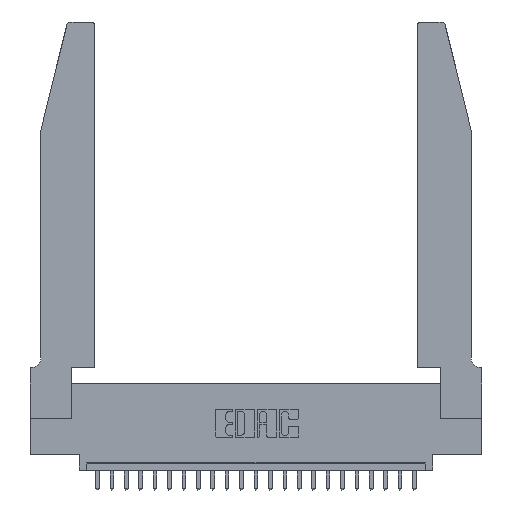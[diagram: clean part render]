
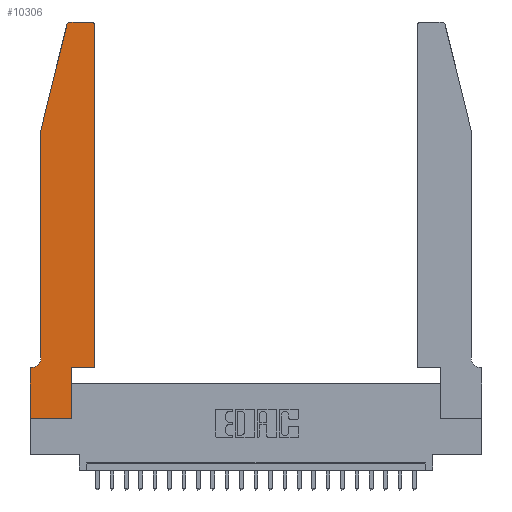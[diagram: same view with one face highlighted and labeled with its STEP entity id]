
A CAD part, top view. The second image highlights one B-rep face of the part: STEP entity #10306.
In plain terms, the highlighted planar face has unit normal (0, 0, 1).
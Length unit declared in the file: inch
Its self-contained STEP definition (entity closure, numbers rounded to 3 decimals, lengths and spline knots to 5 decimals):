
#1007 = CIRCLE ( 'NONE', #1622, 0.03 ) ;
#1274 = CARTESIAN_POINT ( 'NONE',  ( 0.4505, 0.35, 0.37 ) ) ;
#1544 = DIRECTION ( 'NONE',  ( 0., 0., 1. ) ) ;
#1580 = VECTOR ( 'NONE', #18417, 39.37008 ) ;
#1622 = AXIS2_PLACEMENT_3D ( 'NONE', #13395, #7715, #19280 ) ;
#1625 = DIRECTION ( 'NONE',  ( 1., 0., 0. ) ) ;
#1990 = ORIENTED_EDGE ( 'NONE', *, *, #8757, .T. ) ;
#2129 = LINE ( 'NONE', #23747, #23075 ) ;
#2935 = ORIENTED_EDGE ( 'NONE', *, *, #4413, .T. ) ;
#3007 = EDGE_CURVE ( 'NONE', #4921, #15804, #4898, .T. ) ;
#3213 = CARTESIAN_POINT ( 'NONE',  ( 0., 0., 0.37 ) ) ;
#3584 = CARTESIAN_POINT ( 'NONE',  ( 0.284, 2.72, 0.37 ) ) ;
#3932 = VERTEX_POINT ( 'NONE', #20603 ) ;
#4021 = VERTEX_POINT ( 'NONE', #6823 ) ;
#4277 = EDGE_CURVE ( 'NONE', #3932, #5333, #21621, .T. ) ;
#4413 = EDGE_CURVE ( 'NONE', #14375, #3932, #19214, .T. ) ;
#4443 = CARTESIAN_POINT ( 'NONE',  ( 0.0055, 0.35, 0.37 ) ) ;
#4565 = VECTOR ( 'NONE', #5075, 39.37008 ) ;
#4867 = VERTEX_POINT ( 'NONE', #18776 ) ;
#4884 = EDGE_CURVE ( 'NONE', #12663, #22410, #17072, .T. ) ;
#4898 = LINE ( 'NONE', #14768, #4565 ) ;
#4921 = VERTEX_POINT ( 'NONE', #5695 ) ;
#5075 = DIRECTION ( 'NONE',  ( 0., -1., 0. ) ) ;
#5246 = DIRECTION ( 'NONE',  ( 0., 0., -1. ) ) ;
#5313 = EDGE_CURVE ( 'NONE', #5333, #4921, #2129, .T. ) ;
#5333 = VERTEX_POINT ( 'NONE', #9057 ) ;
#5490 = VERTEX_POINT ( 'NONE', #4443 ) ;
#5508 = CARTESIAN_POINT ( 'NONE',  ( 0., 0., 0.37 ) ) ;
#5695 = CARTESIAN_POINT ( 'NONE',  ( 0.0755, 2., 0.37 ) ) ;
#5872 = LINE ( 'NONE', #5508, #15428 ) ;
#6413 = LINE ( 'NONE', #1274, #12709 ) ;
#6823 = CARTESIAN_POINT ( 'NONE',  ( 0.2865, 0.35, 0.37 ) ) ;
#7454 = DIRECTION ( 'NONE',  ( 0., 0., 1. ) ) ;
#7471 = PLANE ( 'NONE',  #10209 ) ;
#7536 = CARTESIAN_POINT ( 'NONE',  ( 0.4505, 0.35, 0.37 ) ) ;
#7715 = DIRECTION ( 'NONE',  ( 0., 0., 1. ) ) ;
#7973 = ORIENTED_EDGE ( 'NONE', *, *, #13818, .T. ) ;
#8038 = CARTESIAN_POINT ( 'NONE',  ( 0.0755, 0.35, 0.37 ) ) ;
#8757 = EDGE_CURVE ( 'NONE', #15804, #5490, #24688, .T. ) ;
#9057 = CARTESIAN_POINT ( 'NONE',  ( 0.25487, 2.72718, 0.37 ) ) ;
#9566 = DIRECTION ( 'NONE',  ( -1., 0., 0. ) ) ;
#10193 = LINE ( 'NONE', #7536, #18278 ) ;
#10209 = AXIS2_PLACEMENT_3D ( 'NONE', #15140, #1544, #1625 ) ;
#10306 = ADVANCED_FACE ( 'NONE', ( #22839 ), #7471, .T. ) ;
#10510 = CARTESIAN_POINT ( 'NONE',  ( 0., 0.35, 0.37 ) ) ;
#10618 = EDGE_CURVE ( 'NONE', #22410, #4021, #22213, .T. ) ;
#10808 = VECTOR ( 'NONE', #9566, 39.37008 ) ;
#11042 = ORIENTED_EDGE ( 'NONE', *, *, #4884, .T. ) ;
#11117 = DIRECTION ( 'NONE',  ( 1., 0., 0. ) ) ;
#11588 = ORIENTED_EDGE ( 'NONE', *, *, #4277, .T. ) ;
#11668 = ORIENTED_EDGE ( 'NONE', *, *, #22695, .T. ) ;
#12079 = VERTEX_POINT ( 'NONE', #10510 ) ;
#12152 = CARTESIAN_POINT ( 'NONE',  ( 0., 0., 0.37 ) ) ;
#12483 = CARTESIAN_POINT ( 'NONE',  ( 0.2865, 0., 0.37 ) ) ;
#12663 = VERTEX_POINT ( 'NONE', #12152 ) ;
#12709 = VECTOR ( 'NONE', #16323, 39.37008 ) ;
#12897 = CARTESIAN_POINT ( 'NONE',  ( 0.4505, 0.35, 0.37 ) ) ;
#13355 = EDGE_LOOP ( 'NONE', ( #2935, #11588, #17117, #16468, #1990, #20863, #7973, #11042, #15535, #14066, #24223, #11668 ) ) ;
#13394 = VERTEX_POINT ( 'NONE', #12897 ) ;
#13395 = CARTESIAN_POINT ( 'NONE',  ( 0.4205, 2.72, 0.37 ) ) ;
#13818 = EDGE_CURVE ( 'NONE', #12079, #12663, #5872, .T. ) ;
#14066 = ORIENTED_EDGE ( 'NONE', *, *, #20459, .T. ) ;
#14361 = EDGE_CURVE ( 'NONE', #5490, #12079, #14854, .T. ) ;
#14375 = VERTEX_POINT ( 'NONE', #19613 ) ;
#14768 = CARTESIAN_POINT ( 'NONE',  ( 0.0755, 2., 0.37 ) ) ;
#14854 = LINE ( 'NONE', #8038, #21784 ) ;
#15140 = CARTESIAN_POINT ( 'NONE',  ( 0., 0.35, 0.37 ) ) ;
#15428 = VECTOR ( 'NONE', #24220, 39.37008 ) ;
#15535 = ORIENTED_EDGE ( 'NONE', *, *, #10618, .T. ) ;
#15804 = VERTEX_POINT ( 'NONE', #18873 ) ;
#15879 = DIRECTION ( 'NONE',  ( -1., 0., 0. ) ) ;
#16323 = DIRECTION ( 'NONE',  ( 0., 1., 0. ) ) ;
#16468 = ORIENTED_EDGE ( 'NONE', *, *, #3007, .T. ) ;
#16491 = VECTOR ( 'NONE', #20910, 39.37008 ) ;
#16680 = CARTESIAN_POINT ( 'NONE',  ( 0.2865, 0.35, 0.37 ) ) ;
#16868 = CARTESIAN_POINT ( 'NONE',  ( 0.0055, 0.42, 0.37 ) ) ;
#17072 = LINE ( 'NONE', #3213, #16491 ) ;
#17117 = ORIENTED_EDGE ( 'NONE', *, *, #5313, .T. ) ;
#17171 = CARTESIAN_POINT ( 'NONE',  ( 0.2605, 2.75, 0.37 ) ) ;
#18170 = EDGE_CURVE ( 'NONE', #13394, #4867, #6413, .T. ) ;
#18278 = VECTOR ( 'NONE', #11117, 39.37008 ) ;
#18417 = DIRECTION ( 'NONE',  ( 0., 1., 0. ) ) ;
#18776 = CARTESIAN_POINT ( 'NONE',  ( 0.4505, 2.72, 0.37 ) ) ;
#18873 = CARTESIAN_POINT ( 'NONE',  ( 0.0755, 0.42, 0.37 ) ) ;
#19098 = DIRECTION ( 'NONE',  ( 1., 0., 0. ) ) ;
#19214 = LINE ( 'NONE', #17171, #10808 ) ;
#19280 = DIRECTION ( 'NONE',  ( 1., 0., 0. ) ) ;
#19300 = AXIS2_PLACEMENT_3D ( 'NONE', #3584, #7454, #19098 ) ;
#19613 = CARTESIAN_POINT ( 'NONE',  ( 0.4205, 2.75, 0.37 ) ) ;
#20459 = EDGE_CURVE ( 'NONE', #4021, #13394, #10193, .T. ) ;
#20543 = DIRECTION ( 'NONE',  ( -0.239, -0.971, 0. ) ) ;
#20603 = CARTESIAN_POINT ( 'NONE',  ( 0.284, 2.75, 0.37 ) ) ;
#20604 = DIRECTION ( 'NONE',  ( -1., 0., 0. ) ) ;
#20863 = ORIENTED_EDGE ( 'NONE', *, *, #14361, .T. ) ;
#20910 = DIRECTION ( 'NONE',  ( 1., 0., 0. ) ) ;
#21621 = CIRCLE ( 'NONE', #19300, 0.03 ) ;
#21784 = VECTOR ( 'NONE', #15879, 39.37008 ) ;
#22213 = LINE ( 'NONE', #16680, #1580 ) ;
#22410 = VERTEX_POINT ( 'NONE', #12483 ) ;
#22695 = EDGE_CURVE ( 'NONE', #4867, #14375, #1007, .T. ) ;
#22839 = FACE_OUTER_BOUND ( 'NONE', #13355, .T. ) ;
#23075 = VECTOR ( 'NONE', #20543, 39.37008 ) ;
#23747 = CARTESIAN_POINT ( 'NONE',  ( 0.0755, 2., 0.37 ) ) ;
#24220 = DIRECTION ( 'NONE',  ( 0., -1., 0. ) ) ;
#24223 = ORIENTED_EDGE ( 'NONE', *, *, #18170, .T. ) ;
#24287 = AXIS2_PLACEMENT_3D ( 'NONE', #16868, #5246, #20604 ) ;
#24688 = CIRCLE ( 'NONE', #24287, 0.07 ) ;
